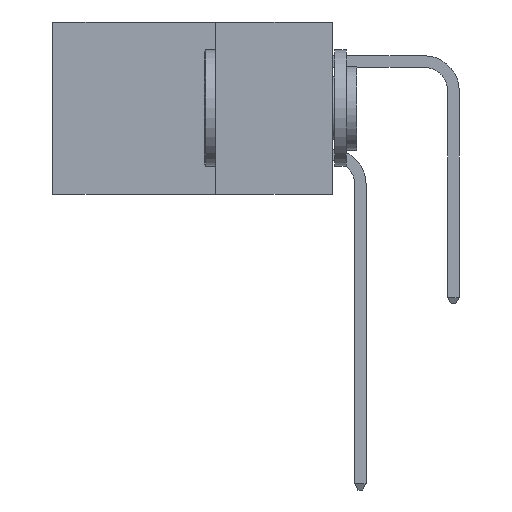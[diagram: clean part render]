
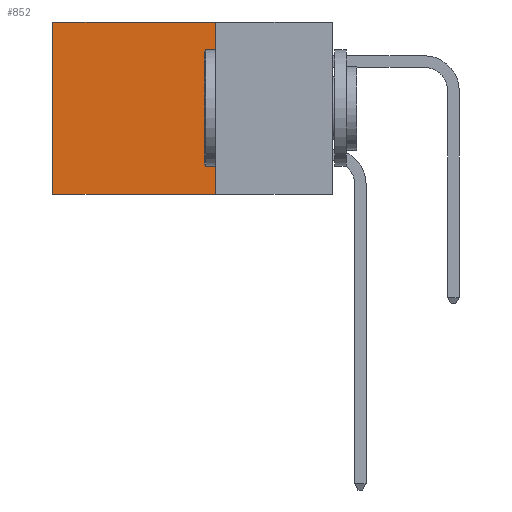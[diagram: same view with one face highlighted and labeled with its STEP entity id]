
A CAD part, left-side view. The second image highlights one B-rep face of the part: STEP entity #852.
In plain terms, the highlighted planar face has unit normal (-1, 0, 0).
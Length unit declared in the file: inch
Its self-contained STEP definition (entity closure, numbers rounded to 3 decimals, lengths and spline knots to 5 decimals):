
#423 = LINE ( 'NONE', #9733, #12837 ) ;
#643 = EDGE_CURVE ( 'NONE', #9563, #7962, #11159, .T. ) ;
#852 = ADVANCED_FACE ( 'NONE', ( #5470 ), #3487, .F. ) ;
#1856 = CARTESIAN_POINT ( 'NONE',  ( 0.2615, 0.25, -0.37 ) ) ;
#2427 = CARTESIAN_POINT ( 'NONE',  ( 0.2615, 0.6, -0.37 ) ) ;
#3097 = VECTOR ( 'NONE', #12142, 39.37008 ) ;
#3204 = EDGE_CURVE ( 'NONE', #12482, #9563, #10970, .T. ) ;
#3420 = CARTESIAN_POINT ( 'NONE',  ( 0.2615, 0.25, -0.37 ) ) ;
#3487 = PLANE ( 'NONE',  #8643 ) ;
#3534 = VERTEX_POINT ( 'NONE', #9590 ) ;
#4299 = DIRECTION ( 'NONE',  ( 1., 0., 0. ) ) ;
#4788 = CARTESIAN_POINT ( 'NONE',  ( 0.2615, 0.25, -0.37 ) ) ;
#5470 = FACE_OUTER_BOUND ( 'NONE', #11140, .T. ) ;
#6173 = ORIENTED_EDGE ( 'NONE', *, *, #7487, .T. ) ;
#6218 = ORIENTED_EDGE ( 'NONE', *, *, #643, .F. ) ;
#6339 = ORIENTED_EDGE ( 'NONE', *, *, #3204, .F. ) ;
#6396 = VECTOR ( 'NONE', #8575, 39.37008 ) ;
#7235 = CARTESIAN_POINT ( 'NONE',  ( 0.2615, 0.6, -0.37 ) ) ;
#7487 = EDGE_CURVE ( 'NONE', #3534, #7962, #8997, .T. ) ;
#7641 = EDGE_CURVE ( 'NONE', #12482, #3534, #423, .T. ) ;
#7821 = DIRECTION ( 'NONE',  ( 0., 1., 0. ) ) ;
#7829 = ORIENTED_EDGE ( 'NONE', *, *, #7641, .T. ) ;
#7919 = DIRECTION ( 'NONE',  ( 0., 0., -1. ) ) ;
#7962 = VERTEX_POINT ( 'NONE', #7235 ) ;
#8335 = VECTOR ( 'NONE', #12859, 39.37008 ) ;
#8575 = DIRECTION ( 'NONE',  ( 0., 0., -1. ) ) ;
#8643 = AXIS2_PLACEMENT_3D ( 'NONE', #3420, #4299, #7919 ) ;
#8997 = LINE ( 'NONE', #2427, #6396 ) ;
#9563 = VERTEX_POINT ( 'NONE', #4788 ) ;
#9590 = CARTESIAN_POINT ( 'NONE',  ( 0.2615, 0.6, 0. ) ) ;
#9733 = CARTESIAN_POINT ( 'NONE',  ( 0.2615, 0.25, 0. ) ) ;
#10970 = LINE ( 'NONE', #11538, #3097 ) ;
#11140 = EDGE_LOOP ( 'NONE', ( #6173, #6218, #6339, #7829 ) ) ;
#11159 = LINE ( 'NONE', #1856, #8335 ) ;
#11538 = CARTESIAN_POINT ( 'NONE',  ( 0.2615, 0.25, -0.37 ) ) ;
#12142 = DIRECTION ( 'NONE',  ( 0., 0., -1. ) ) ;
#12163 = CARTESIAN_POINT ( 'NONE',  ( 0.2615, 0.25, 0. ) ) ;
#12482 = VERTEX_POINT ( 'NONE', #12163 ) ;
#12837 = VECTOR ( 'NONE', #7821, 39.37008 ) ;
#12859 = DIRECTION ( 'NONE',  ( 0., 1., 0. ) ) ;
